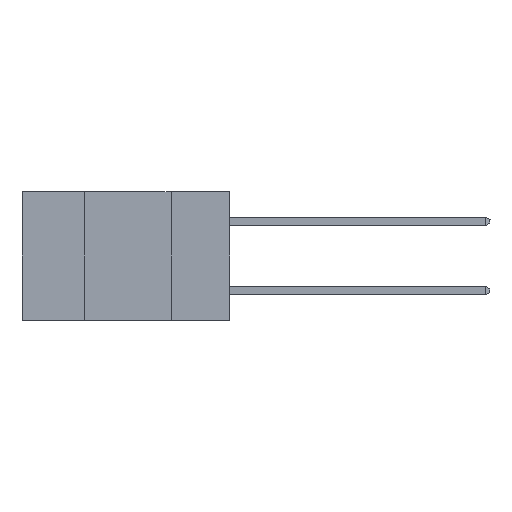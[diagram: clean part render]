
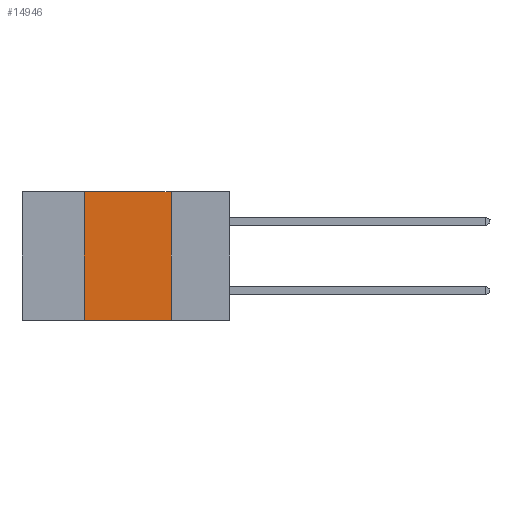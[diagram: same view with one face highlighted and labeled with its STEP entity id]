
A CAD part, left-side view. The second image highlights one B-rep face of the part: STEP entity #14946.
In plain terms, the highlighted planar face has unit normal (-1, 0, 0).
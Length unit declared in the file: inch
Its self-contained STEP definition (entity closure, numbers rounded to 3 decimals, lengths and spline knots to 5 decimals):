
#358 = ORIENTED_EDGE ( 'NONE', *, *, #17371, .F. ) ;
#548 = PLANE ( 'NONE',  #16038 ) ;
#899 = CARTESIAN_POINT ( 'NONE',  ( 0., 0.17, 0. ) ) ;
#1025 = VERTEX_POINT ( 'NONE', #17911 ) ;
#1718 = CARTESIAN_POINT ( 'NONE',  ( 0., 0.17, -0.37 ) ) ;
#2197 = DIRECTION ( 'NONE',  ( 0., 0., -1. ) ) ;
#3041 = LINE ( 'NONE', #16064, #11301 ) ;
#3792 = CARTESIAN_POINT ( 'NONE',  ( 0., 0.6, 0. ) ) ;
#5123 = LINE ( 'NONE', #21034, #13385 ) ;
#5552 = DIRECTION ( 'NONE',  ( 0., 0., -1. ) ) ;
#7987 = VERTEX_POINT ( 'NONE', #899 ) ;
#8046 = LINE ( 'NONE', #8228, #16196 ) ;
#8165 = VECTOR ( 'NONE', #5552, 39.37008 ) ;
#8228 = CARTESIAN_POINT ( 'NONE',  ( 0., 0.6, -0.37 ) ) ;
#8542 = EDGE_CURVE ( 'NONE', #7987, #9035, #16822, .T. ) ;
#9035 = VERTEX_POINT ( 'NONE', #1718 ) ;
#9678 = CARTESIAN_POINT ( 'NONE',  ( 0., 0.42, 0. ) ) ;
#9701 = EDGE_LOOP ( 'NONE', ( #13486, #358, #12960, #10666 ) ) ;
#9850 = DIRECTION ( 'NONE',  ( 0., -1., 0. ) ) ;
#10436 = FACE_OUTER_BOUND ( 'NONE', #9701, .T. ) ;
#10666 = ORIENTED_EDGE ( 'NONE', *, *, #16160, .T. ) ;
#11301 = VECTOR ( 'NONE', #19204, 39.37008 ) ;
#12008 = VERTEX_POINT ( 'NONE', #9678 ) ;
#12069 = DIRECTION ( 'NONE',  ( 1., 0., 0. ) ) ;
#12109 = CARTESIAN_POINT ( 'NONE',  ( 0., 0.17, 0. ) ) ;
#12960 = ORIENTED_EDGE ( 'NONE', *, *, #17931, .F. ) ;
#13230 = DIRECTION ( 'NONE',  ( 0., -1., 0. ) ) ;
#13385 = VECTOR ( 'NONE', #9850, 39.37008 ) ;
#13486 = ORIENTED_EDGE ( 'NONE', *, *, #8542, .F. ) ;
#14946 = ADVANCED_FACE ( 'NONE', ( #10436 ), #548, .F. ) ;
#16038 = AXIS2_PLACEMENT_3D ( 'NONE', #3792, #12069, #2197 ) ;
#16064 = CARTESIAN_POINT ( 'NONE',  ( 0., 0.42, 0. ) ) ;
#16160 = EDGE_CURVE ( 'NONE', #1025, #9035, #8046, .T. ) ;
#16196 = VECTOR ( 'NONE', #13230, 39.37008 ) ;
#16822 = LINE ( 'NONE', #12109, #8165 ) ;
#17371 = EDGE_CURVE ( 'NONE', #12008, #7987, #5123, .T. ) ;
#17911 = CARTESIAN_POINT ( 'NONE',  ( 0., 0.42, -0.37 ) ) ;
#17931 = EDGE_CURVE ( 'NONE', #1025, #12008, #3041, .T. ) ;
#19204 = DIRECTION ( 'NONE',  ( 0., 0., 1. ) ) ;
#21034 = CARTESIAN_POINT ( 'NONE',  ( 0., 0.6, 0. ) ) ;
